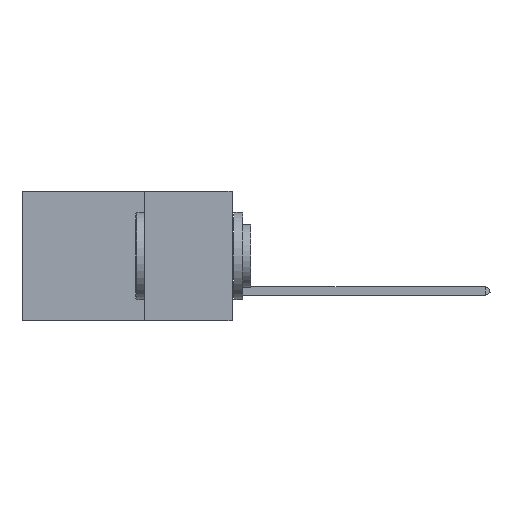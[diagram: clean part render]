
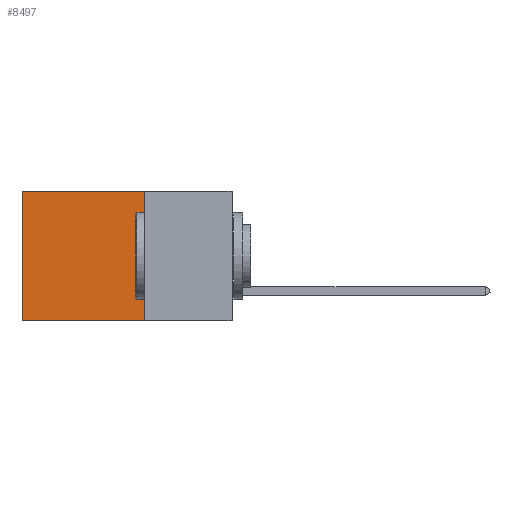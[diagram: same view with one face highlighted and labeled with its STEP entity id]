
A CAD part, left-side view. The second image highlights one B-rep face of the part: STEP entity #8497.
In plain terms, the highlighted planar face has unit normal (-1, 0, 0).
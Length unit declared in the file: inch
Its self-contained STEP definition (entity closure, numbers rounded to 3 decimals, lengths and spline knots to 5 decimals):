
#332 = DIRECTION ( 'NONE',  ( 0., 1., 0. ) ) ;
#1164 = DIRECTION ( 'NONE',  ( 1., 0., 0. ) ) ;
#1479 = ORIENTED_EDGE ( 'NONE', *, *, #8038, .T. ) ;
#1666 = VERTEX_POINT ( 'NONE', #2076 ) ;
#2024 = EDGE_CURVE ( 'NONE', #1666, #8131, #10779, .T. ) ;
#2076 = CARTESIAN_POINT ( 'NONE',  ( 0.2875, 0.25, 0. ) ) ;
#2408 = DIRECTION ( 'NONE',  ( 0., 0., -1. ) ) ;
#2710 = ORIENTED_EDGE ( 'NONE', *, *, #2024, .T. ) ;
#3585 = VECTOR ( 'NONE', #332, 39.37008 ) ;
#4127 = CARTESIAN_POINT ( 'NONE',  ( 0.2875, 0.25, -0.37 ) ) ;
#4128 = VECTOR ( 'NONE', #9094, 39.37008 ) ;
#4744 = LINE ( 'NONE', #13087, #6753 ) ;
#4798 = FACE_OUTER_BOUND ( 'NONE', #7588, .T. ) ;
#5406 = CARTESIAN_POINT ( 'NONE',  ( 0.2875, 0.25, -0.37 ) ) ;
#6391 = VERTEX_POINT ( 'NONE', #4127 ) ;
#6753 = VECTOR ( 'NONE', #7156, 39.37008 ) ;
#7156 = DIRECTION ( 'NONE',  ( 0., 0., -1. ) ) ;
#7319 = CARTESIAN_POINT ( 'NONE',  ( 0.2875, 0.25, 0. ) ) ;
#7588 = EDGE_LOOP ( 'NONE', ( #1479, #9543, #11335, #2710 ) ) ;
#7785 = CARTESIAN_POINT ( 'NONE',  ( 0.2875, 0.6, 0. ) ) ;
#7884 = CARTESIAN_POINT ( 'NONE',  ( 0.2875, 0.6, -0.37 ) ) ;
#8038 = EDGE_CURVE ( 'NONE', #8131, #8149, #9915, .T. ) ;
#8131 = VERTEX_POINT ( 'NONE', #12709 ) ;
#8149 = VERTEX_POINT ( 'NONE', #7884 ) ;
#8497 = ADVANCED_FACE ( 'NONE', ( #4798 ), #12964, .F. ) ;
#8846 = EDGE_CURVE ( 'NONE', #1666, #6391, #4744, .T. ) ;
#9094 = DIRECTION ( 'NONE',  ( 0., 1., 0. ) ) ;
#9543 = ORIENTED_EDGE ( 'NONE', *, *, #9964, .F. ) ;
#9915 = LINE ( 'NONE', #7785, #12325 ) ;
#9964 = EDGE_CURVE ( 'NONE', #6391, #8149, #13762, .T. ) ;
#10050 = AXIS2_PLACEMENT_3D ( 'NONE', #14171, #1164, #2408 ) ;
#10779 = LINE ( 'NONE', #7319, #3585 ) ;
#11335 = ORIENTED_EDGE ( 'NONE', *, *, #8846, .F. ) ;
#12325 = VECTOR ( 'NONE', #12336, 39.37008 ) ;
#12336 = DIRECTION ( 'NONE',  ( 0., 0., -1. ) ) ;
#12709 = CARTESIAN_POINT ( 'NONE',  ( 0.2875, 0.6, 0. ) ) ;
#12964 = PLANE ( 'NONE',  #10050 ) ;
#13087 = CARTESIAN_POINT ( 'NONE',  ( 0.2875, 0.25, 0. ) ) ;
#13762 = LINE ( 'NONE', #5406, #4128 ) ;
#14171 = CARTESIAN_POINT ( 'NONE',  ( 0.2875, 0.25, 0. ) ) ;
